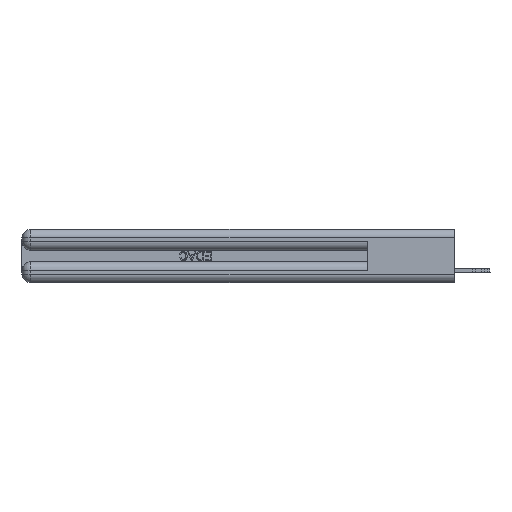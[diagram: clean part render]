
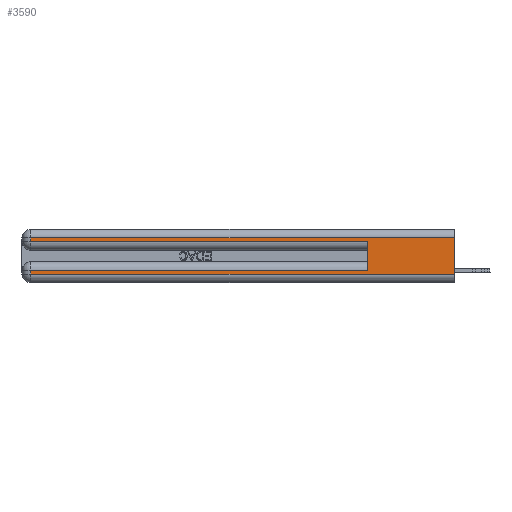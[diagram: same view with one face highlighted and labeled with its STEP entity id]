
A CAD part, left-side view. The second image highlights one B-rep face of the part: STEP entity #3590.
In plain terms, the highlighted planar face has unit normal (-1, 0, 0).
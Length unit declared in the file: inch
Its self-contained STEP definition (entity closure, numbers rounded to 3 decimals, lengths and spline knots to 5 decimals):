
#518 = LINE ( 'NONE', #7105, #1878 ) ;
#1811 = CARTESIAN_POINT ( 'NONE',  ( 0., 0.6, 0.285 ) ) ;
#1878 = VECTOR ( 'NONE', #36849, 39.37008 ) ;
#2143 = ORIENTED_EDGE ( 'NONE', *, *, #51670, .T. ) ;
#2999 = VECTOR ( 'NONE', #8980, 39.37008 ) ;
#3590 = ADVANCED_FACE ( 'NONE', ( #24462 ), #35885, .F. ) ;
#3668 = VERTEX_POINT ( 'NONE', #23499 ) ;
#5651 = DIRECTION ( 'NONE',  ( 0., -1., 0. ) ) ;
#6213 = VERTEX_POINT ( 'NONE', #44514 ) ;
#7105 = CARTESIAN_POINT ( 'NONE',  ( 0., 0., 0.31 ) ) ;
#7541 = ORIENTED_EDGE ( 'NONE', *, *, #40828, .T. ) ;
#7754 = VECTOR ( 'NONE', #20623, 39.37008 ) ;
#8001 = CARTESIAN_POINT ( 'NONE',  ( 0., 0., 0.06 ) ) ;
#8980 = DIRECTION ( 'NONE',  ( 0., 0., -1. ) ) ;
#9178 = EDGE_CURVE ( 'NONE', #33063, #27798, #22465, .T. ) ;
#9345 = VERTEX_POINT ( 'NONE', #15958 ) ;
#12283 = EDGE_CURVE ( 'NONE', #9345, #37606, #23504, .T. ) ;
#13279 = CARTESIAN_POINT ( 'NONE',  ( 0., 2.94, 0.37 ) ) ;
#15107 = EDGE_CURVE ( 'NONE', #6213, #3668, #518, .T. ) ;
#15135 = CARTESIAN_POINT ( 'NONE',  ( 0., 0.6, 0.085 ) ) ;
#15958 = CARTESIAN_POINT ( 'NONE',  ( 0., 2.94, 0.06 ) ) ;
#16362 = ORIENTED_EDGE ( 'NONE', *, *, #12283, .T. ) ;
#16918 = CARTESIAN_POINT ( 'NONE',  ( 0., 0., 0.06 ) ) ;
#17429 = EDGE_LOOP ( 'NONE', ( #48708, #23289, #7541, #30799, #43503, #2143, #25317, #16362 ) ) ;
#19073 = AXIS2_PLACEMENT_3D ( 'NONE', #23133, #19331, #39533 ) ;
#19331 = DIRECTION ( 'NONE',  ( 1., 0., 0. ) ) ;
#20520 = CARTESIAN_POINT ( 'NONE',  ( 0., 0., 0.085 ) ) ;
#20623 = DIRECTION ( 'NONE',  ( 0., 0., 1. ) ) ;
#21100 = EDGE_CURVE ( 'NONE', #6213, #37606, #48797, .T. ) ;
#21264 = DIRECTION ( 'NONE',  ( 0., 0., -1. ) ) ;
#21751 = CARTESIAN_POINT ( 'NONE',  ( 0., 2.94, 0.085 ) ) ;
#22465 = LINE ( 'NONE', #28361, #7754 ) ;
#23133 = CARTESIAN_POINT ( 'NONE',  ( 0., 0., 0.37 ) ) ;
#23253 = EDGE_CURVE ( 'NONE', #52736, #27798, #42565, .T. ) ;
#23289 = ORIENTED_EDGE ( 'NONE', *, *, #15107, .T. ) ;
#23499 = CARTESIAN_POINT ( 'NONE',  ( 0., 2.94, 0.31 ) ) ;
#23504 = LINE ( 'NONE', #8001, #37619 ) ;
#24462 = FACE_OUTER_BOUND ( 'NONE', #17429, .T. ) ;
#25317 = ORIENTED_EDGE ( 'NONE', *, *, #28223, .T. ) ;
#25644 = DIRECTION ( 'NONE',  ( 0., 0., -1. ) ) ;
#27798 = VERTEX_POINT ( 'NONE', #1811 ) ;
#28223 = EDGE_CURVE ( 'NONE', #29954, #9345, #48280, .T. ) ;
#28357 = VECTOR ( 'NONE', #21264, 39.37008 ) ;
#28361 = CARTESIAN_POINT ( 'NONE',  ( 0., 0.6, 0.145 ) ) ;
#28683 = CARTESIAN_POINT ( 'NONE',  ( 0., 2.94, 0.285 ) ) ;
#29431 = CARTESIAN_POINT ( 'NONE',  ( 0., 2.94, 0.37 ) ) ;
#29954 = VERTEX_POINT ( 'NONE', #21751 ) ;
#30705 = VECTOR ( 'NONE', #25644, 39.37008 ) ;
#30799 = ORIENTED_EDGE ( 'NONE', *, *, #23253, .T. ) ;
#31772 = VECTOR ( 'NONE', #5651, 39.37008 ) ;
#32723 = LINE ( 'NONE', #29431, #2999 ) ;
#33063 = VERTEX_POINT ( 'NONE', #15135 ) ;
#33370 = DIRECTION ( 'NONE',  ( 0., 1., 0. ) ) ;
#35885 = PLANE ( 'NONE',  #19073 ) ;
#36849 = DIRECTION ( 'NONE',  ( 0., 1., 0. ) ) ;
#37606 = VERTEX_POINT ( 'NONE', #16918 ) ;
#37619 = VECTOR ( 'NONE', #40963, 39.37008 ) ;
#38998 = CARTESIAN_POINT ( 'NONE',  ( 0., 0., 0.285 ) ) ;
#39533 = DIRECTION ( 'NONE',  ( 0., 0., -1. ) ) ;
#40828 = EDGE_CURVE ( 'NONE', #3668, #52736, #32723, .T. ) ;
#40963 = DIRECTION ( 'NONE',  ( 0., -1., 0. ) ) ;
#41523 = CARTESIAN_POINT ( 'NONE',  ( 0., 0., 0.37 ) ) ;
#42565 = LINE ( 'NONE', #38998, #31772 ) ;
#43503 = ORIENTED_EDGE ( 'NONE', *, *, #9178, .F. ) ;
#44514 = CARTESIAN_POINT ( 'NONE',  ( 0., 0., 0.31 ) ) ;
#45862 = VECTOR ( 'NONE', #33370, 39.37008 ) ;
#47154 = LINE ( 'NONE', #20520, #45862 ) ;
#48280 = LINE ( 'NONE', #13279, #28357 ) ;
#48708 = ORIENTED_EDGE ( 'NONE', *, *, #21100, .F. ) ;
#48797 = LINE ( 'NONE', #41523, #30705 ) ;
#51670 = EDGE_CURVE ( 'NONE', #33063, #29954, #47154, .T. ) ;
#52736 = VERTEX_POINT ( 'NONE', #28683 ) ;
